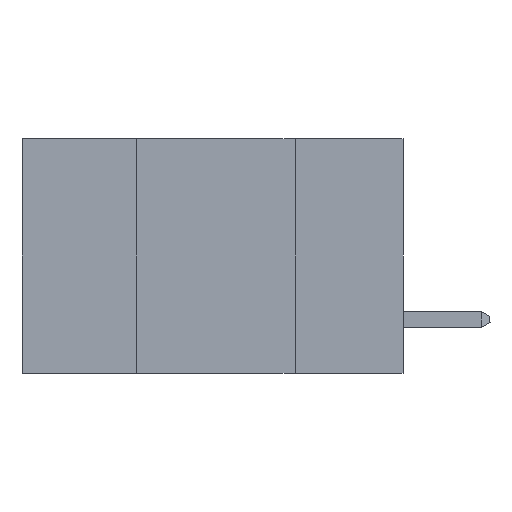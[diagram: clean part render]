
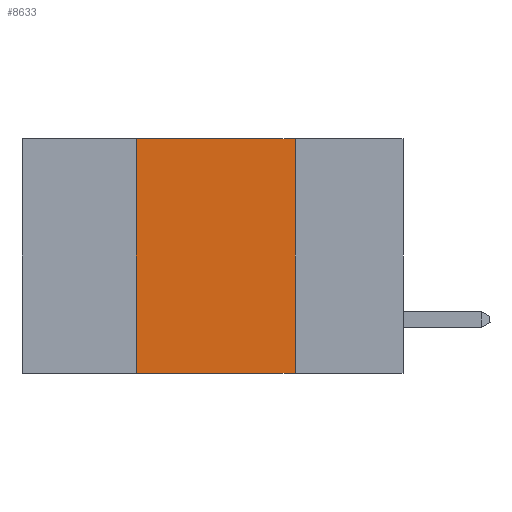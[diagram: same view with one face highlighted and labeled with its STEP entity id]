
A CAD part, left-side view. The second image highlights one B-rep face of the part: STEP entity #8633.
In plain terms, the highlighted planar face has unit normal (-1, 0, 0).
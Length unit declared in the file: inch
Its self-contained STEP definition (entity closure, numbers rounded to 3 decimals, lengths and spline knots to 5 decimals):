
#1026 = CARTESIAN_POINT ( 'NONE',  ( 0., 0.6, -0.37 ) ) ;
#1090 = EDGE_CURVE ( 'NONE', #9079, #14616, #12588, .T. ) ;
#1142 = PLANE ( 'NONE',  #7718 ) ;
#1326 = VERTEX_POINT ( 'NONE', #12974 ) ;
#1620 = FACE_OUTER_BOUND ( 'NONE', #4155, .T. ) ;
#2615 = VERTEX_POINT ( 'NONE', #4390 ) ;
#2828 = CARTESIAN_POINT ( 'NONE',  ( 0., 0.42, -0.37 ) ) ;
#3305 = VECTOR ( 'NONE', #9745, 39.37008 ) ;
#3698 = VECTOR ( 'NONE', #11968, 39.37008 ) ;
#4041 = VECTOR ( 'NONE', #10219, 39.37008 ) ;
#4081 = LINE ( 'NONE', #7011, #3698 ) ;
#4155 = EDGE_LOOP ( 'NONE', ( #13932, #12047, #8258, #13915 ) ) ;
#4390 = CARTESIAN_POINT ( 'NONE',  ( 0., 0.42, 0. ) ) ;
#5817 = CARTESIAN_POINT ( 'NONE',  ( 0., 0.6, 0. ) ) ;
#7011 = CARTESIAN_POINT ( 'NONE',  ( 0., 0.6, 0. ) ) ;
#7038 = EDGE_CURVE ( 'NONE', #2615, #1326, #4081, .T. ) ;
#7718 = AXIS2_PLACEMENT_3D ( 'NONE', #5817, #13973, #9200 ) ;
#7816 = EDGE_CURVE ( 'NONE', #1326, #14616, #8570, .T. ) ;
#8258 = ORIENTED_EDGE ( 'NONE', *, *, #13150, .F. ) ;
#8434 = CARTESIAN_POINT ( 'NONE',  ( 0., 0.17, -0.37 ) ) ;
#8570 = LINE ( 'NONE', #13396, #10448 ) ;
#8633 = ADVANCED_FACE ( 'NONE', ( #1620 ), #1142, .F. ) ;
#8916 = LINE ( 'NONE', #12981, #3305 ) ;
#9079 = VERTEX_POINT ( 'NONE', #2828 ) ;
#9200 = DIRECTION ( 'NONE',  ( 0., 0., -1. ) ) ;
#9745 = DIRECTION ( 'NONE',  ( 0., 0., 1. ) ) ;
#10219 = DIRECTION ( 'NONE',  ( 0., -1., 0. ) ) ;
#10448 = VECTOR ( 'NONE', #10977, 39.37008 ) ;
#10977 = DIRECTION ( 'NONE',  ( 0., 0., -1. ) ) ;
#11968 = DIRECTION ( 'NONE',  ( 0., -1., 0. ) ) ;
#12047 = ORIENTED_EDGE ( 'NONE', *, *, #7038, .F. ) ;
#12588 = LINE ( 'NONE', #1026, #4041 ) ;
#12974 = CARTESIAN_POINT ( 'NONE',  ( 0., 0.17, 0. ) ) ;
#12981 = CARTESIAN_POINT ( 'NONE',  ( 0., 0.42, 0. ) ) ;
#13150 = EDGE_CURVE ( 'NONE', #9079, #2615, #8916, .T. ) ;
#13396 = CARTESIAN_POINT ( 'NONE',  ( 0., 0.17, 0. ) ) ;
#13915 = ORIENTED_EDGE ( 'NONE', *, *, #1090, .T. ) ;
#13932 = ORIENTED_EDGE ( 'NONE', *, *, #7816, .F. ) ;
#13973 = DIRECTION ( 'NONE',  ( 1., 0., 0. ) ) ;
#14616 = VERTEX_POINT ( 'NONE', #8434 ) ;
